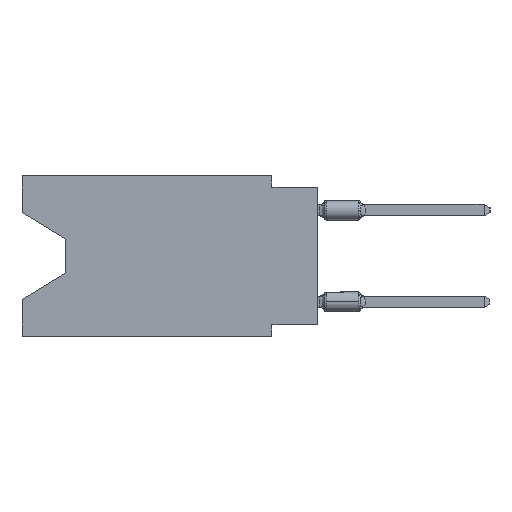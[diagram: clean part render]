
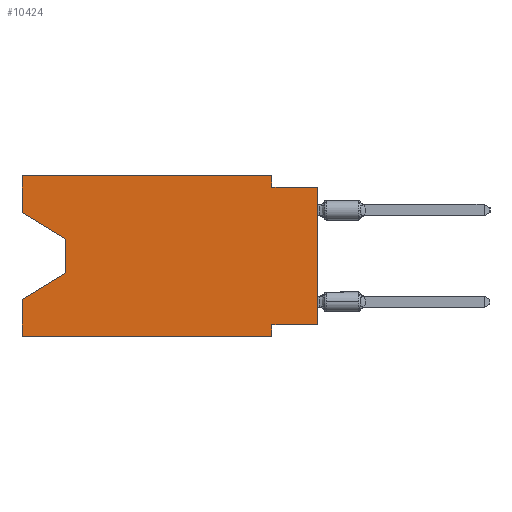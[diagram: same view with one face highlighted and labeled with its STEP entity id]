
A CAD part, left-side view. The second image highlights one B-rep face of the part: STEP entity #10424.
In plain terms, the highlighted planar face has unit normal (-1, 0, 0).
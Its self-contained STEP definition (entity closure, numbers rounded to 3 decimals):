
#247 = CARTESIAN_POINT ( 'NONE',  ( 0., 16.383, 0. ) ) ;
#1153 = EDGE_LOOP ( 'NONE', ( #34097, #46883, #27094, #50178, #46492, #6572, #16339, #46964, #48595, #6132, #52242, #21113 ) ) ;
#2272 = VERTEX_POINT ( 'NONE', #10445 ) ;
#2984 = DIRECTION ( 'NONE',  ( 0., -1., 0. ) ) ;
#3525 = CARTESIAN_POINT ( 'NONE',  ( 0., 2.54, 0. ) ) ;
#3563 = EDGE_CURVE ( 'NONE', #16097, #9323, #54693, .T. ) ;
#3659 = DIRECTION ( 'NONE',  ( 0., 0., -1. ) ) ;
#4865 = LINE ( 'NONE', #43032, #6452 ) ;
#4957 = CARTESIAN_POINT ( 'NONE',  ( 0., 16.383, -2.038 ) ) ;
#5195 = CARTESIAN_POINT ( 'NONE',  ( 0., 2.54, -8.255 ) ) ;
#5272 = CARTESIAN_POINT ( 'NONE',  ( 0., 2.54, 0. ) ) ;
#6132 = ORIENTED_EDGE ( 'NONE', *, *, #3563, .F. ) ;
#6330 = EDGE_CURVE ( 'NONE', #43427, #40597, #36271, .T. ) ;
#6452 = VECTOR ( 'NONE', #17055, 1000. ) ;
#6572 = ORIENTED_EDGE ( 'NONE', *, *, #45647, .F. ) ;
#9072 = CARTESIAN_POINT ( 'NONE',  ( 0., 16.383, 0. ) ) ;
#9323 = VERTEX_POINT ( 'NONE', #47085 ) ;
#10424 = ADVANCED_FACE ( 'NONE', ( #22939 ), #39819, .F. ) ;
#10445 = CARTESIAN_POINT ( 'NONE',  ( 0., 0., -0.635 ) ) ;
#11559 = DIRECTION ( 'NONE',  ( 0., 0., -1. ) ) ;
#12054 = DIRECTION ( 'NONE',  ( 0., 0.855, -0.519 ) ) ;
#12846 = VECTOR ( 'NONE', #12054, 1000. ) ;
#14829 = EDGE_CURVE ( 'NONE', #50887, #46820, #50356, .T. ) ;
#15198 = DIRECTION ( 'NONE',  ( 0., 0., -1. ) ) ;
#15569 = LINE ( 'NONE', #32155, #22557 ) ;
#15772 = CARTESIAN_POINT ( 'NONE',  ( 0., 0., 0. ) ) ;
#16097 = VERTEX_POINT ( 'NONE', #5272 ) ;
#16339 = ORIENTED_EDGE ( 'NONE', *, *, #6330, .F. ) ;
#17055 = DIRECTION ( 'NONE',  ( 0., 0., -1. ) ) ;
#17389 = LINE ( 'NONE', #9072, #54089 ) ;
#17500 = VERTEX_POINT ( 'NONE', #19113 ) ;
#18508 = CARTESIAN_POINT ( 'NONE',  ( 0., 16.383, 0. ) ) ;
#18786 = DIRECTION ( 'NONE',  ( 1., 0., 0. ) ) ;
#19113 = CARTESIAN_POINT ( 'NONE',  ( 0., 13.97, -5.385 ) ) ;
#19576 = VECTOR ( 'NONE', #29543, 1000. ) ;
#19627 = LINE ( 'NONE', #15772, #24411 ) ;
#21113 = ORIENTED_EDGE ( 'NONE', *, *, #33054, .F. ) ;
#21252 = VECTOR ( 'NONE', #3659, 1000. ) ;
#21980 = CARTESIAN_POINT ( 'NONE',  ( 0., 16.383, 0. ) ) ;
#22557 = VECTOR ( 'NONE', #24125, 1000. ) ;
#22618 = DIRECTION ( 'NONE',  ( 0., -1., 0. ) ) ;
#22939 = FACE_OUTER_BOUND ( 'NONE', #1153, .T. ) ;
#23052 = EDGE_CURVE ( 'NONE', #43427, #2272, #19627, .T. ) ;
#24125 = DIRECTION ( 'NONE',  ( 0., -1., 0. ) ) ;
#24153 = LINE ( 'NONE', #53485, #21252 ) ;
#24411 = VECTOR ( 'NONE', #36507, 1000. ) ;
#25318 = CARTESIAN_POINT ( 'NONE',  ( 0., 13.97, -3.505 ) ) ;
#26388 = DIRECTION ( 'NONE',  ( 0., 0., 1. ) ) ;
#27094 = ORIENTED_EDGE ( 'NONE', *, *, #52401, .T. ) ;
#27325 = CARTESIAN_POINT ( 'NONE',  ( 0., 16.383, -8.89 ) ) ;
#29543 = DIRECTION ( 'NONE',  ( 0., 0., 1. ) ) ;
#29770 = EDGE_CURVE ( 'NONE', #9323, #2272, #15569, .T. ) ;
#31674 = VECTOR ( 'NONE', #42334, 1000. ) ;
#32155 = CARTESIAN_POINT ( 'NONE',  ( 0., 0., -0.635 ) ) ;
#33054 = EDGE_CURVE ( 'NONE', #50887, #50331, #54723, .T. ) ;
#33723 = CARTESIAN_POINT ( 'NONE',  ( 0., 16.383, -8.89 ) ) ;
#34097 = ORIENTED_EDGE ( 'NONE', *, *, #14829, .T. ) ;
#36271 = LINE ( 'NONE', #48449, #47814 ) ;
#36454 = LINE ( 'NONE', #27325, #46882 ) ;
#36507 = DIRECTION ( 'NONE',  ( 0., 0., 1. ) ) ;
#36567 = CARTESIAN_POINT ( 'NONE',  ( 0., 16.383, 0. ) ) ;
#37440 = EDGE_CURVE ( 'NONE', #44120, #51523, #39129, .T. ) ;
#37899 = CARTESIAN_POINT ( 'NONE',  ( 0., 16.383, -6.852 ) ) ;
#39129 = LINE ( 'NONE', #21980, #43628 ) ;
#39374 = EDGE_CURVE ( 'NONE', #50331, #16097, #17389, .T. ) ;
#39377 = CARTESIAN_POINT ( 'NONE',  ( 0., 0., -8.255 ) ) ;
#39819 = PLANE ( 'NONE',  #49924 ) ;
#39872 = DIRECTION ( 'NONE',  ( 0., 1., 0. ) ) ;
#40597 = VERTEX_POINT ( 'NONE', #5195 ) ;
#41642 = CARTESIAN_POINT ( 'NONE',  ( 0., 13.97, -5.385 ) ) ;
#42334 = DIRECTION ( 'NONE',  ( 0., -0.855, -0.519 ) ) ;
#43032 = CARTESIAN_POINT ( 'NONE',  ( 0., 2.54, -8.89 ) ) ;
#43381 = CARTESIAN_POINT ( 'NONE',  ( 0., 2.54, -8.89 ) ) ;
#43427 = VERTEX_POINT ( 'NONE', #39377 ) ;
#43628 = VECTOR ( 'NONE', #26388, 1000. ) ;
#44120 = VERTEX_POINT ( 'NONE', #33723 ) ;
#44349 = EDGE_CURVE ( 'NONE', #44120, #50536, #36454, .T. ) ;
#45647 = EDGE_CURVE ( 'NONE', #40597, #50536, #4865, .T. ) ;
#46492 = ORIENTED_EDGE ( 'NONE', *, *, #44349, .T. ) ;
#46820 = VERTEX_POINT ( 'NONE', #25318 ) ;
#46882 = VECTOR ( 'NONE', #2984, 1000. ) ;
#46883 = ORIENTED_EDGE ( 'NONE', *, *, #49816, .T. ) ;
#46964 = ORIENTED_EDGE ( 'NONE', *, *, #23052, .T. ) ;
#47085 = CARTESIAN_POINT ( 'NONE',  ( 0., 2.54, -0.635 ) ) ;
#47814 = VECTOR ( 'NONE', #39872, 1000. ) ;
#48443 = VECTOR ( 'NONE', #11559, 1000. ) ;
#48449 = CARTESIAN_POINT ( 'NONE',  ( 0., 0., -8.255 ) ) ;
#48595 = ORIENTED_EDGE ( 'NONE', *, *, #29770, .F. ) ;
#49816 = EDGE_CURVE ( 'NONE', #46820, #17500, #24153, .T. ) ;
#49924 = AXIS2_PLACEMENT_3D ( 'NONE', #18508, #18786, #15198 ) ;
#49956 = LINE ( 'NONE', #41642, #12846 ) ;
#50178 = ORIENTED_EDGE ( 'NONE', *, *, #37440, .F. ) ;
#50331 = VERTEX_POINT ( 'NONE', #247 ) ;
#50356 = LINE ( 'NONE', #4957, #31674 ) ;
#50536 = VERTEX_POINT ( 'NONE', #43381 ) ;
#50887 = VERTEX_POINT ( 'NONE', #52379 ) ;
#51523 = VERTEX_POINT ( 'NONE', #37899 ) ;
#52242 = ORIENTED_EDGE ( 'NONE', *, *, #39374, .F. ) ;
#52379 = CARTESIAN_POINT ( 'NONE',  ( 0., 16.383, -2.038 ) ) ;
#52401 = EDGE_CURVE ( 'NONE', #17500, #51523, #49956, .T. ) ;
#53485 = CARTESIAN_POINT ( 'NONE',  ( 0., 13.97, -3.505 ) ) ;
#54089 = VECTOR ( 'NONE', #22618, 1000. ) ;
#54693 = LINE ( 'NONE', #3525, #48443 ) ;
#54723 = LINE ( 'NONE', #36567, #19576 ) ;
